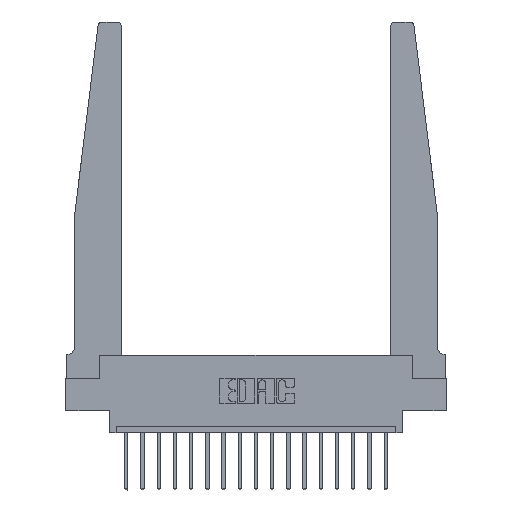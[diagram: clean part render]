
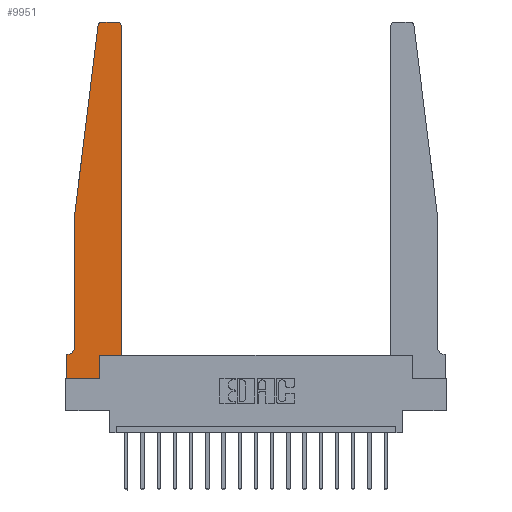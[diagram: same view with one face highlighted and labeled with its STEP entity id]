
A CAD part, top view. The second image highlights one B-rep face of the part: STEP entity #9951.
In plain terms, the highlighted planar face has unit normal (0, 0, 1).
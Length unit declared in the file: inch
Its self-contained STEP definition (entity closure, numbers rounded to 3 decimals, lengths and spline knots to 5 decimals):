
#276 = AXIS2_PLACEMENT_3D ( 'NONE', #2940, #12912, #13385 ) ;
#278 = CARTESIAN_POINT ( 'NONE',  ( 0.425, 0.18, 0.37 ) ) ;
#302 = AXIS2_PLACEMENT_3D ( 'NONE', #544, #2102, #15464 ) ;
#541 = CARTESIAN_POINT ( 'NONE',  ( 0., 0., 0.37 ) ) ;
#544 = CARTESIAN_POINT ( 'NONE',  ( 0., 0.1875, 0.37 ) ) ;
#650 = DIRECTION ( 'NONE',  ( 0., 0., 1. ) ) ;
#804 = VECTOR ( 'NONE', #18454, 39.37008 ) ;
#1156 = VECTOR ( 'NONE', #11962, 39.37008 ) ;
#1273 = DIRECTION ( 'NONE',  ( 0., 1., 0. ) ) ;
#1442 = VERTEX_POINT ( 'NONE', #6315 ) ;
#1534 = CARTESIAN_POINT ( 'NONE',  ( 0.065, 1.25, 0.37 ) ) ;
#1889 = CARTESIAN_POINT ( 'NONE',  ( 0.425, 0.18, 0.37 ) ) ;
#2102 = DIRECTION ( 'NONE',  ( 0., 0., 1. ) ) ;
#2106 = VERTEX_POINT ( 'NONE', #17955 ) ;
#2150 = DIRECTION ( 'NONE',  ( -1., 0., 0. ) ) ;
#2268 = EDGE_CURVE ( 'NONE', #15000, #7208, #8657, .T. ) ;
#2329 = VECTOR ( 'NONE', #1273, 39.37008 ) ;
#2333 = CARTESIAN_POINT ( 'NONE',  ( 0.015, 0.2375, 0.37 ) ) ;
#2672 = LINE ( 'NONE', #14865, #12362 ) ;
#2681 = ORIENTED_EDGE ( 'NONE', *, *, #9912, .T. ) ;
#2718 = DIRECTION ( 'NONE',  ( -1., 0., 0. ) ) ;
#2940 = CARTESIAN_POINT ( 'NONE',  ( 0.395, 2.72, 0.37 ) ) ;
#3356 = ORIENTED_EDGE ( 'NONE', *, *, #6984, .T. ) ;
#3389 = EDGE_CURVE ( 'NONE', #10602, #15305, #16877, .T. ) ;
#3394 = ORIENTED_EDGE ( 'NONE', *, *, #10456, .T. ) ;
#3634 = CARTESIAN_POINT ( 'NONE',  ( 0.425, 0.18, 0.37 ) ) ;
#3671 = CARTESIAN_POINT ( 'NONE',  ( 0., 0., 0.37 ) ) ;
#4020 = VECTOR ( 'NONE', #14373, 39.37008 ) ;
#4657 = ORIENTED_EDGE ( 'NONE', *, *, #7237, .T. ) ;
#4718 = EDGE_CURVE ( 'NONE', #10168, #16808, #10123, .T. ) ;
#4989 = ORIENTED_EDGE ( 'NONE', *, *, #10709, .T. ) ;
#5211 = PLANE ( 'NONE',  #302 ) ;
#5232 = AXIS2_PLACEMENT_3D ( 'NONE', #2333, #5646, #2718 ) ;
#5488 = ORIENTED_EDGE ( 'NONE', *, *, #8879, .T. ) ;
#5571 = LINE ( 'NONE', #11520, #17942 ) ;
#5646 = DIRECTION ( 'NONE',  ( 0., 0., -1. ) ) ;
#5785 = EDGE_CURVE ( 'NONE', #12210, #17674, #15545, .T. ) ;
#5854 = CARTESIAN_POINT ( 'NONE',  ( 0.425, 2.72, 0.37 ) ) ;
#6315 = CARTESIAN_POINT ( 'NONE',  ( 0.2605, 0.18, 0.37 ) ) ;
#6367 = CARTESIAN_POINT ( 'NONE',  ( 0.2605, 0.18, 0.37 ) ) ;
#6558 = ORIENTED_EDGE ( 'NONE', *, *, #3389, .T. ) ;
#6590 = CARTESIAN_POINT ( 'NONE',  ( 0.24675, 2.72367, 0.37 ) ) ;
#6705 = LINE ( 'NONE', #3671, #18925 ) ;
#6984 = EDGE_CURVE ( 'NONE', #2106, #1442, #17818, .T. ) ;
#7062 = CARTESIAN_POINT ( 'NONE',  ( 0.065, 0.2375, 0.37 ) ) ;
#7208 = VERTEX_POINT ( 'NONE', #8782 ) ;
#7237 = EDGE_CURVE ( 'NONE', #8819, #2106, #2672, .T. ) ;
#7694 = CARTESIAN_POINT ( 'NONE',  ( 0.27653, 2.75, 0.37 ) ) ;
#7875 = CARTESIAN_POINT ( 'NONE',  ( 0.25, 2.75, 0.37 ) ) ;
#8328 = CIRCLE ( 'NONE', #276, 0.03 ) ;
#8555 = CARTESIAN_POINT ( 'NONE',  ( 0.065, 0.1875, 0.37 ) ) ;
#8657 = LINE ( 'NONE', #8555, #4020 ) ;
#8668 = ORIENTED_EDGE ( 'NONE', *, *, #4718, .T. ) ;
#8736 = CARTESIAN_POINT ( 'NONE',  ( 0.395, 2.75, 0.37 ) ) ;
#8782 = CARTESIAN_POINT ( 'NONE',  ( 0., 0.1875, 0.37 ) ) ;
#8819 = VERTEX_POINT ( 'NONE', #541 ) ;
#8879 = EDGE_CURVE ( 'NONE', #16808, #10602, #8328, .T. ) ;
#9912 = EDGE_CURVE ( 'NONE', #15305, #12034, #15874, .T. ) ;
#9951 = ADVANCED_FACE ( 'NONE', ( #18565 ), #5211, .T. ) ;
#10123 = LINE ( 'NONE', #3634, #2329 ) ;
#10168 = VERTEX_POINT ( 'NONE', #1889 ) ;
#10246 = EDGE_LOOP ( 'NONE', ( #6558, #2681, #12996, #12826, #3394, #17263, #15482, #4657, #3356, #4989, #8668, #5488 ) ) ;
#10456 = EDGE_CURVE ( 'NONE', #17674, #15000, #13982, .T. ) ;
#10602 = VERTEX_POINT ( 'NONE', #8736 ) ;
#10709 = EDGE_CURVE ( 'NONE', #1442, #10168, #12356, .T. ) ;
#10873 = CARTESIAN_POINT ( 'NONE',  ( 0.27653, 2.72, 0.37 ) ) ;
#11244 = CARTESIAN_POINT ( 'NONE',  ( 0.015, 0.1875, 0.37 ) ) ;
#11328 = VECTOR ( 'NONE', #2150, 39.37008 ) ;
#11417 = DIRECTION ( 'NONE',  ( -0.122, -0.992, 0. ) ) ;
#11520 = CARTESIAN_POINT ( 'NONE',  ( 0.065, 1.25, 0.37 ) ) ;
#11962 = DIRECTION ( 'NONE',  ( 0., 1., 0. ) ) ;
#12034 = VERTEX_POINT ( 'NONE', #6590 ) ;
#12210 = VERTEX_POINT ( 'NONE', #1534 ) ;
#12356 = LINE ( 'NONE', #278, #18312 ) ;
#12362 = VECTOR ( 'NONE', #13407, 39.37008 ) ;
#12757 = AXIS2_PLACEMENT_3D ( 'NONE', #10873, #650, #15659 ) ;
#12826 = ORIENTED_EDGE ( 'NONE', *, *, #5785, .T. ) ;
#12912 = DIRECTION ( 'NONE',  ( 0., 0., 1. ) ) ;
#12996 = ORIENTED_EDGE ( 'NONE', *, *, #16679, .T. ) ;
#13385 = DIRECTION ( 'NONE',  ( 1., 0., 0. ) ) ;
#13407 = DIRECTION ( 'NONE',  ( 1., 0., 0. ) ) ;
#13982 = CIRCLE ( 'NONE', #5232, 0.05 ) ;
#14373 = DIRECTION ( 'NONE',  ( -1., 0., 0. ) ) ;
#14865 = CARTESIAN_POINT ( 'NONE',  ( 0., 0., 0.37 ) ) ;
#15000 = VERTEX_POINT ( 'NONE', #11244 ) ;
#15305 = VERTEX_POINT ( 'NONE', #7694 ) ;
#15381 = DIRECTION ( 'NONE',  ( 0., -1., 0. ) ) ;
#15385 = DIRECTION ( 'NONE',  ( 1., 0., 0. ) ) ;
#15464 = DIRECTION ( 'NONE',  ( 1., 0., 0. ) ) ;
#15482 = ORIENTED_EDGE ( 'NONE', *, *, #18415, .T. ) ;
#15545 = LINE ( 'NONE', #18361, #804 ) ;
#15659 = DIRECTION ( 'NONE',  ( 1., 0., 0. ) ) ;
#15874 = CIRCLE ( 'NONE', #12757, 0.03 ) ;
#16679 = EDGE_CURVE ( 'NONE', #12034, #12210, #5571, .T. ) ;
#16808 = VERTEX_POINT ( 'NONE', #5854 ) ;
#16877 = LINE ( 'NONE', #7875, #11328 ) ;
#17263 = ORIENTED_EDGE ( 'NONE', *, *, #2268, .T. ) ;
#17674 = VERTEX_POINT ( 'NONE', #7062 ) ;
#17818 = LINE ( 'NONE', #6367, #1156 ) ;
#17942 = VECTOR ( 'NONE', #11417, 39.37008 ) ;
#17955 = CARTESIAN_POINT ( 'NONE',  ( 0.2605, 0., 0.37 ) ) ;
#18312 = VECTOR ( 'NONE', #15385, 39.37008 ) ;
#18361 = CARTESIAN_POINT ( 'NONE',  ( 0.065, 1.25, 0.37 ) ) ;
#18415 = EDGE_CURVE ( 'NONE', #7208, #8819, #6705, .T. ) ;
#18454 = DIRECTION ( 'NONE',  ( 0., -1., 0. ) ) ;
#18565 = FACE_OUTER_BOUND ( 'NONE', #10246, .T. ) ;
#18925 = VECTOR ( 'NONE', #15381, 39.37008 ) ;
